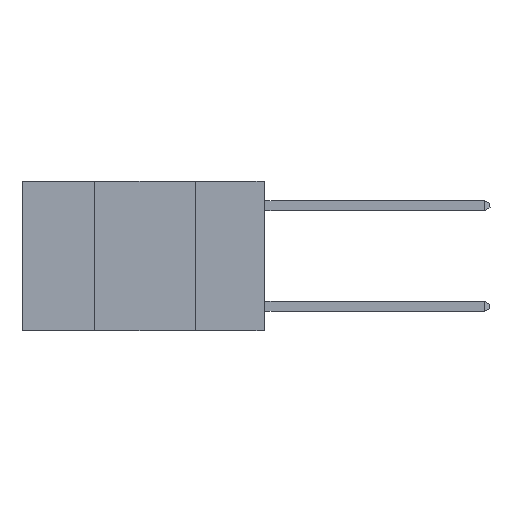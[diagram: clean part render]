
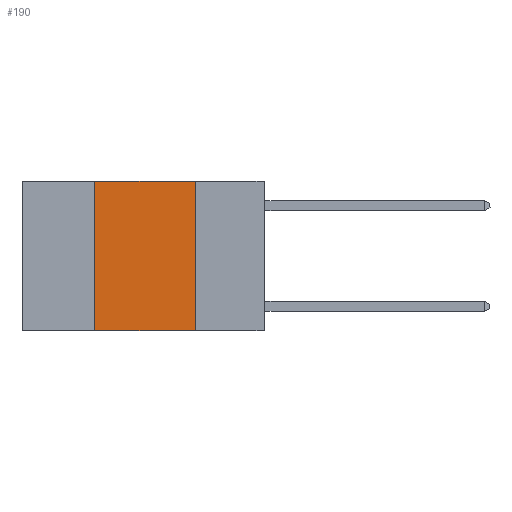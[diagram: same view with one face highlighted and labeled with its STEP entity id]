
A CAD part, left-side view. The second image highlights one B-rep face of the part: STEP entity #190.
In plain terms, the highlighted planar face has unit normal (-1, 0, 0).
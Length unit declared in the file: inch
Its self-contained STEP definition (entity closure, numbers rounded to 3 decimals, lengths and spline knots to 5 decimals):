
#190 = ADVANCED_FACE ( 'NONE', ( #761 ), #3477, .F. ) ;
#201 = DIRECTION ( 'NONE',  ( 0., -1., 0. ) ) ;
#303 = VERTEX_POINT ( 'NONE', #4910 ) ;
#311 = VECTOR ( 'NONE', #5883, 39.37008 ) ;
#345 = EDGE_LOOP ( 'NONE', ( #1608, #6517, #3273, #2969 ) ) ;
#478 = DIRECTION ( 'NONE',  ( 1., 0., 0. ) ) ;
#505 = CARTESIAN_POINT ( 'NONE',  ( 0., 0.17, 0. ) ) ;
#680 = EDGE_CURVE ( 'NONE', #6728, #303, #6028, .T. ) ;
#761 = FACE_OUTER_BOUND ( 'NONE', #345, .T. ) ;
#832 = CARTESIAN_POINT ( 'NONE',  ( 0., 0.42, -0.37 ) ) ;
#1031 = EDGE_CURVE ( 'NONE', #303, #4497, #1917, .T. ) ;
#1608 = ORIENTED_EDGE ( 'NONE', *, *, #2038, .F. ) ;
#1744 = LINE ( 'NONE', #7580, #5308 ) ;
#1901 = VECTOR ( 'NONE', #6429, 39.37008 ) ;
#1917 = LINE ( 'NONE', #4751, #5801 ) ;
#2038 = EDGE_CURVE ( 'NONE', #4497, #8060, #3875, .T. ) ;
#2580 = DIRECTION ( 'NONE',  ( 0., -1., 0. ) ) ;
#2770 = CARTESIAN_POINT ( 'NONE',  ( 0., 0.6, 0. ) ) ;
#2969 = ORIENTED_EDGE ( 'NONE', *, *, #3898, .T. ) ;
#3103 = CARTESIAN_POINT ( 'NONE',  ( 0., 0.17, 0. ) ) ;
#3273 = ORIENTED_EDGE ( 'NONE', *, *, #680, .F. ) ;
#3477 = PLANE ( 'NONE',  #4522 ) ;
#3875 = LINE ( 'NONE', #505, #1901 ) ;
#3898 = EDGE_CURVE ( 'NONE', #6728, #8060, #1744, .T. ) ;
#4497 = VERTEX_POINT ( 'NONE', #3103 ) ;
#4522 = AXIS2_PLACEMENT_3D ( 'NONE', #2770, #478, #6788 ) ;
#4751 = CARTESIAN_POINT ( 'NONE',  ( 0., 0.6, 0. ) ) ;
#4910 = CARTESIAN_POINT ( 'NONE',  ( 0., 0.42, 0. ) ) ;
#5308 = VECTOR ( 'NONE', #2580, 39.37008 ) ;
#5801 = VECTOR ( 'NONE', #201, 39.37008 ) ;
#5883 = DIRECTION ( 'NONE',  ( 0., 0., 1. ) ) ;
#6028 = LINE ( 'NONE', #6368, #311 ) ;
#6368 = CARTESIAN_POINT ( 'NONE',  ( 0., 0.42, 0. ) ) ;
#6429 = DIRECTION ( 'NONE',  ( 0., 0., -1. ) ) ;
#6517 = ORIENTED_EDGE ( 'NONE', *, *, #1031, .F. ) ;
#6728 = VERTEX_POINT ( 'NONE', #832 ) ;
#6788 = DIRECTION ( 'NONE',  ( 0., 0., -1. ) ) ;
#7580 = CARTESIAN_POINT ( 'NONE',  ( 0., 0.6, -0.37 ) ) ;
#7756 = CARTESIAN_POINT ( 'NONE',  ( 0., 0.17, -0.37 ) ) ;
#8060 = VERTEX_POINT ( 'NONE', #7756 ) ;
